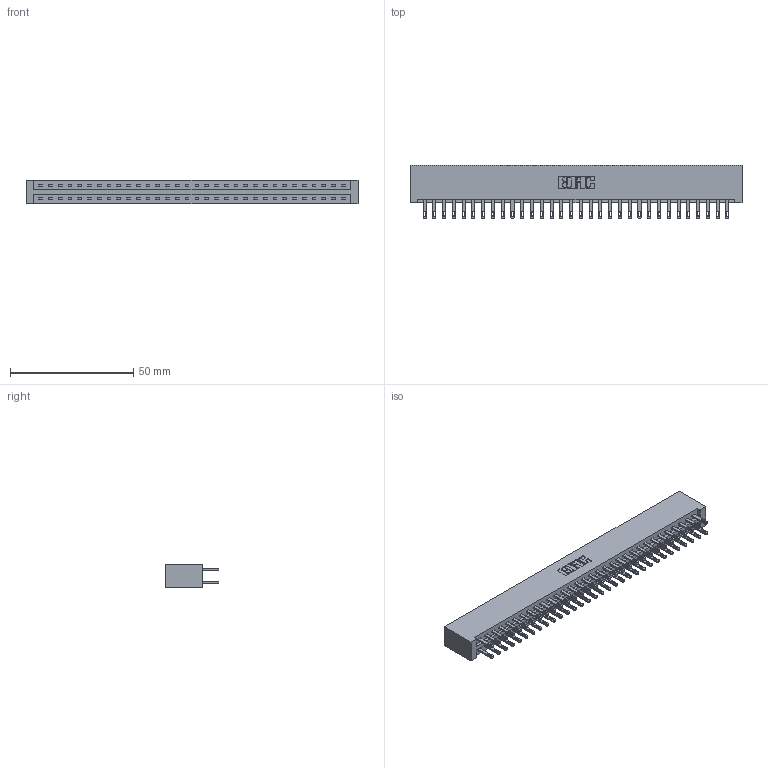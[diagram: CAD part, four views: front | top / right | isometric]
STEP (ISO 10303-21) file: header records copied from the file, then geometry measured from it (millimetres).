
FILE_DESCRIPTION (( 'STEP AP203' ), '1' );
FILE_NAME ('887-064-500-201.STEP', '2020-09-21T02:28:53', ( '' ), ( '' ), 'SwSTEP 2.0', 'SolidWorks 2020', '' );
FILE_SCHEMA (( 'CONFIG_CONTROL_DESIGN' ));
Length unit declared in the file: inch
Products named in the file (3): 887-064-500-201; 345-292-001_345-293-100; 837 Part_No Mounting Lugs
Assembly tree (65 placements, depth 2):
  887-064-500-201
    837 Part_No Mounting Lugs
    345-292-001_345-293-100  x64
Bounding box: 134.67 x 21.85 x 9.4 mm (x, y, z)
Volume: 15015.9 mm3; surface area: 17644.6 mm2
Topology: 65 solids, 65 shells, 3306 faces, 10079 edges, 6718 vertices
Faces by surface type: plane 2114, cylinder 1192
Entity records: 25757 total; most frequent: CARTESIAN_POINT 4346, ORIENTED_EDGE 4282, DIRECTION 3709, EDGE_CURVE 2141, LINE 2017, VECTOR 2017, VERTEX_POINT 1426, AXIS2_PLACEMENT_3D 846
